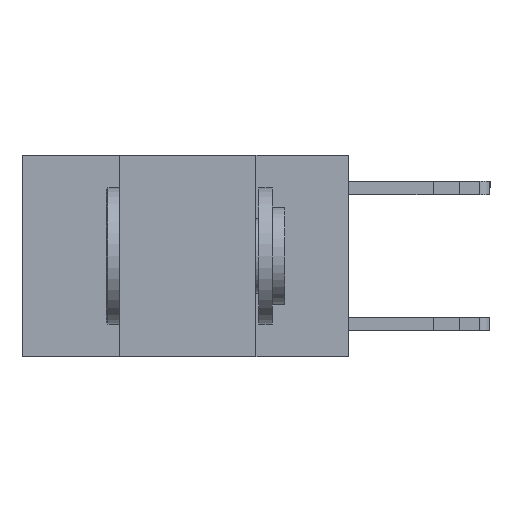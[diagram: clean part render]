
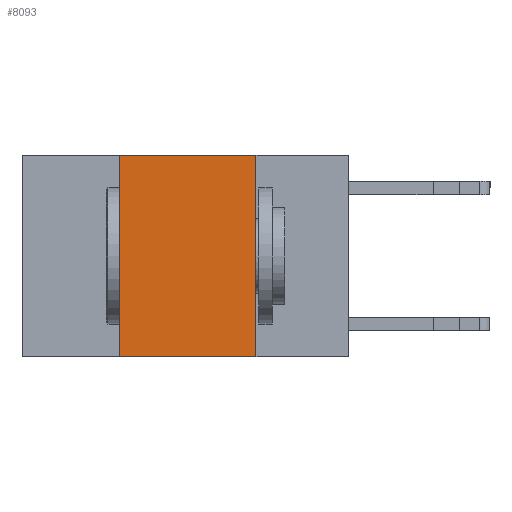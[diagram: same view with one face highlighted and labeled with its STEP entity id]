
A CAD part, left-side view. The second image highlights one B-rep face of the part: STEP entity #8093.
In plain terms, the highlighted planar face has unit normal (-1, 0, 0).
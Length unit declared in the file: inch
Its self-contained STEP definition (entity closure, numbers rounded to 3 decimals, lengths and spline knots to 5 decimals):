
#196 = ORIENTED_EDGE ( 'NONE', *, *, #8911, .F. ) ;
#606 = LINE ( 'NONE', #3781, #5072 ) ;
#656 = CARTESIAN_POINT ( 'NONE',  ( 0., 0.6, 0. ) ) ;
#1062 = CARTESIAN_POINT ( 'NONE',  ( 0., 0.17, 0. ) ) ;
#1135 = LINE ( 'NONE', #12669, #7138 ) ;
#2130 = PLANE ( 'NONE',  #7445 ) ;
#2258 = VERTEX_POINT ( 'NONE', #8059 ) ;
#2696 = VERTEX_POINT ( 'NONE', #9369 ) ;
#3781 = CARTESIAN_POINT ( 'NONE',  ( 0., 0.17, 0. ) ) ;
#4418 = VECTOR ( 'NONE', #7956, 39.37008 ) ;
#5072 = VECTOR ( 'NONE', #13037, 39.37008 ) ;
#6757 = EDGE_CURVE ( 'NONE', #2696, #14370, #10123, .T. ) ;
#6933 = ORIENTED_EDGE ( 'NONE', *, *, #13606, .T. ) ;
#7138 = VECTOR ( 'NONE', #9012, 39.37008 ) ;
#7445 = AXIS2_PLACEMENT_3D ( 'NONE', #656, #9725, #10990 ) ;
#7564 = FACE_OUTER_BOUND ( 'NONE', #14083, .T. ) ;
#7956 = DIRECTION ( 'NONE',  ( 0., -1., 0. ) ) ;
#8059 = CARTESIAN_POINT ( 'NONE',  ( 0., 0.42, -0.37 ) ) ;
#8093 = ADVANCED_FACE ( 'NONE', ( #7564 ), #2130, .F. ) ;
#8449 = VECTOR ( 'NONE', #12211, 39.37008 ) ;
#8911 = EDGE_CURVE ( 'NONE', #14370, #9470, #606, .T. ) ;
#9012 = DIRECTION ( 'NONE',  ( 0., 0., 1. ) ) ;
#9369 = CARTESIAN_POINT ( 'NONE',  ( 0., 0.42, 0. ) ) ;
#9470 = VERTEX_POINT ( 'NONE', #9797 ) ;
#9725 = DIRECTION ( 'NONE',  ( 1., 0., 0. ) ) ;
#9797 = CARTESIAN_POINT ( 'NONE',  ( 0., 0.17, -0.37 ) ) ;
#10041 = LINE ( 'NONE', #12589, #4418 ) ;
#10123 = LINE ( 'NONE', #11172, #8449 ) ;
#10508 = ORIENTED_EDGE ( 'NONE', *, *, #6757, .F. ) ;
#10990 = DIRECTION ( 'NONE',  ( 0., 0., -1. ) ) ;
#11172 = CARTESIAN_POINT ( 'NONE',  ( 0., 0.6, 0. ) ) ;
#11457 = ORIENTED_EDGE ( 'NONE', *, *, #13267, .F. ) ;
#12211 = DIRECTION ( 'NONE',  ( 0., -1., 0. ) ) ;
#12589 = CARTESIAN_POINT ( 'NONE',  ( 0., 0.6, -0.37 ) ) ;
#12669 = CARTESIAN_POINT ( 'NONE',  ( 0., 0.42, 0. ) ) ;
#13037 = DIRECTION ( 'NONE',  ( 0., 0., -1. ) ) ;
#13267 = EDGE_CURVE ( 'NONE', #2258, #2696, #1135, .T. ) ;
#13606 = EDGE_CURVE ( 'NONE', #2258, #9470, #10041, .T. ) ;
#14083 = EDGE_LOOP ( 'NONE', ( #196, #10508, #11457, #6933 ) ) ;
#14370 = VERTEX_POINT ( 'NONE', #1062 ) ;
